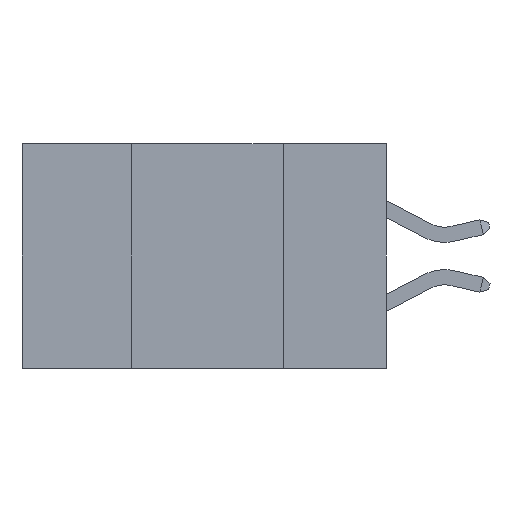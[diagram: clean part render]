
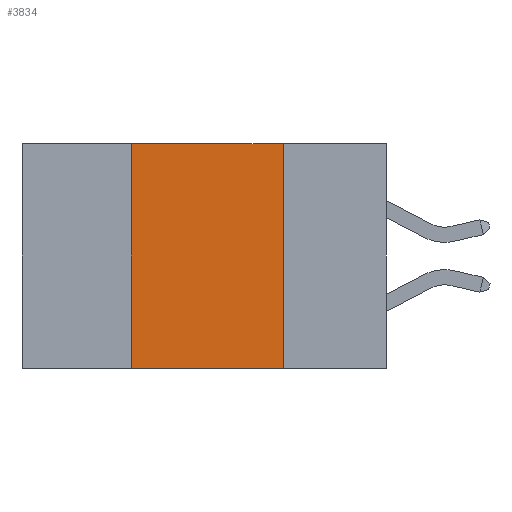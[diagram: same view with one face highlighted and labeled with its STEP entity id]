
A CAD part, left-side view. The second image highlights one B-rep face of the part: STEP entity #3834.
In plain terms, the highlighted planar face has unit normal (-1, 0, 0).
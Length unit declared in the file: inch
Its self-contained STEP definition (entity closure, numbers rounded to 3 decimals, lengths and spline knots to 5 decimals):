
#74 = CARTESIAN_POINT ( 'NONE',  ( 0., 0.42, 0. ) ) ;
#977 = VERTEX_POINT ( 'NONE', #7975 ) ;
#990 = VECTOR ( 'NONE', #11363, 39.37008 ) ;
#1082 = PLANE ( 'NONE',  #5748 ) ;
#1433 = VERTEX_POINT ( 'NONE', #12267 ) ;
#2114 = DIRECTION ( 'NONE',  ( 0., 0., -1. ) ) ;
#2403 = LINE ( 'NONE', #11234, #9950 ) ;
#2489 = DIRECTION ( 'NONE',  ( 0., 0., -1. ) ) ;
#2761 = EDGE_CURVE ( 'NONE', #1433, #5895, #5163, .T. ) ;
#3450 = EDGE_CURVE ( 'NONE', #1433, #9892, #10841, .T. ) ;
#3834 = ADVANCED_FACE ( 'NONE', ( #4911 ), #1082, .F. ) ;
#3871 = CARTESIAN_POINT ( 'NONE',  ( 0., 0.17, -0.37 ) ) ;
#4021 = VECTOR ( 'NONE', #2489, 39.37008 ) ;
#4118 = EDGE_CURVE ( 'NONE', #9892, #977, #2403, .T. ) ;
#4745 = EDGE_CURVE ( 'NONE', #977, #5895, #8907, .T. ) ;
#4911 = FACE_OUTER_BOUND ( 'NONE', #9874, .T. ) ;
#5163 = LINE ( 'NONE', #6313, #7484 ) ;
#5341 = DIRECTION ( 'NONE',  ( 0., -1., 0. ) ) ;
#5575 = CARTESIAN_POINT ( 'NONE',  ( 0., 0.42, -0.37 ) ) ;
#5743 = ORIENTED_EDGE ( 'NONE', *, *, #4745, .F. ) ;
#5748 = AXIS2_PLACEMENT_3D ( 'NONE', #6032, #8043, #2114 ) ;
#5895 = VERTEX_POINT ( 'NONE', #3871 ) ;
#6032 = CARTESIAN_POINT ( 'NONE',  ( 0., 0.6, 0. ) ) ;
#6313 = CARTESIAN_POINT ( 'NONE',  ( 0., 0.6, -0.37 ) ) ;
#7484 = VECTOR ( 'NONE', #5341, 39.37008 ) ;
#7975 = CARTESIAN_POINT ( 'NONE',  ( 0., 0.17, 0. ) ) ;
#8043 = DIRECTION ( 'NONE',  ( 1., 0., 0. ) ) ;
#8685 = ORIENTED_EDGE ( 'NONE', *, *, #4118, .F. ) ;
#8907 = LINE ( 'NONE', #9378, #4021 ) ;
#9302 = ORIENTED_EDGE ( 'NONE', *, *, #2761, .T. ) ;
#9378 = CARTESIAN_POINT ( 'NONE',  ( 0., 0.17, -0.37 ) ) ;
#9383 = DIRECTION ( 'NONE',  ( 0., -1., 0. ) ) ;
#9874 = EDGE_LOOP ( 'NONE', ( #5743, #8685, #11489, #9302 ) ) ;
#9892 = VERTEX_POINT ( 'NONE', #74 ) ;
#9950 = VECTOR ( 'NONE', #9383, 39.37008 ) ;
#10841 = LINE ( 'NONE', #5575, #990 ) ;
#11234 = CARTESIAN_POINT ( 'NONE',  ( 0., 0.6, 0. ) ) ;
#11363 = DIRECTION ( 'NONE',  ( 0., 0., 1. ) ) ;
#11489 = ORIENTED_EDGE ( 'NONE', *, *, #3450, .F. ) ;
#12267 = CARTESIAN_POINT ( 'NONE',  ( 0., 0.42, -0.37 ) ) ;
